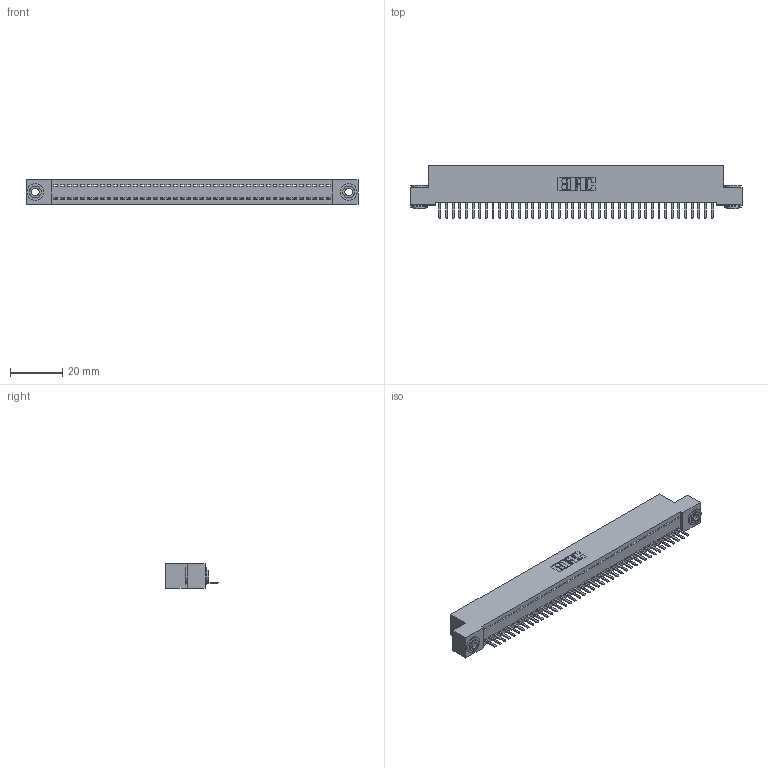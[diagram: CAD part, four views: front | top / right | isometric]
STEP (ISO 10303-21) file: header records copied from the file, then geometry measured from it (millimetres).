
FILE_DESCRIPTION (( 'STEP AP203' ), '1' );
FILE_NAME ('342-042-520-103.STEP', '2018-08-12T02:12:50', ( '' ), ( '' ), 'SwSTEP 2.0', 'SolidWorks 2016', '' );
FILE_SCHEMA (( 'CONFIG_CONTROL_DESIGN' ));
Length unit declared in the file: inch
Products named in the file (4): 342 Part_.156 TH; 345-292-001_345-293-120; 342-250-002_345-250-002-102; 342-042-520-103
Assembly tree (45 placements, depth 2):
  342-042-520-103
    342 Part_.156 TH
    345-292-001_345-293-120  x42
    342-250-002_345-250-002-102  x2
Bounding box: 127 x 20.02 x 9.4 mm (x, y, z)
Volume: 11037.4 mm3; surface area: 16047.6 mm2
Topology: 45 solids, 45 shells, 2752 faces, 8103 edges, 5286 vertices
Faces by surface type: plane 1924, cylinder 820, cone 8
Entity records: 26308 total; most frequent: CARTESIAN_POINT 4527, ORIENTED_EDGE 4486, DIRECTION 3841, EDGE_CURVE 2243, VECTOR 2087, LINE 2087, VERTEX_POINT 1490, AXIS2_PLACEMENT_3D 877
